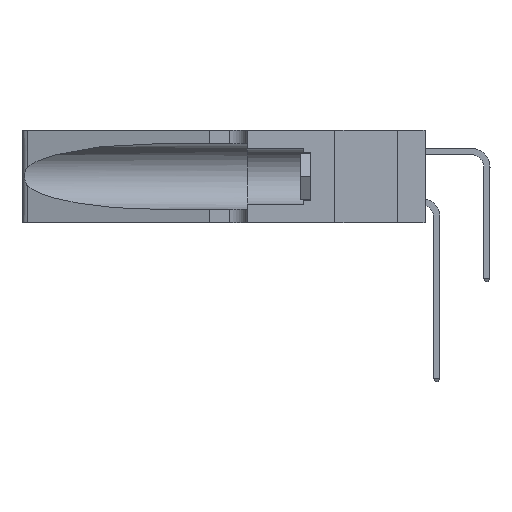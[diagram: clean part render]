
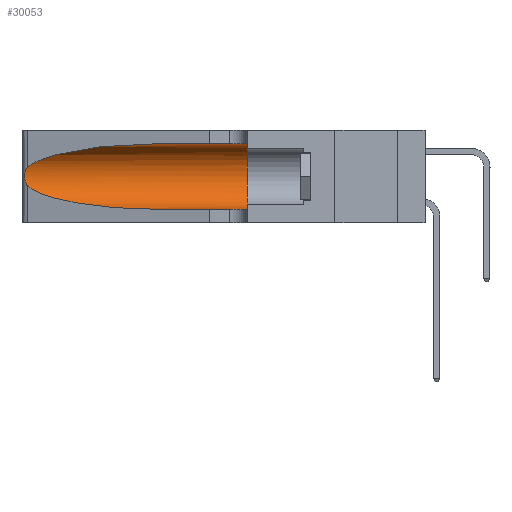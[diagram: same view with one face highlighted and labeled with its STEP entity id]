
A CAD part, left-side view. The second image highlights one B-rep face of the part: STEP entity #30053.
In plain terms, the highlighted cylindrical face has radius 3.308 mm (diameter 6.617 mm), a partial arc.
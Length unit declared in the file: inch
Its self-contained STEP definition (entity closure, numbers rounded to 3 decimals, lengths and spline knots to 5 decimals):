
#41 = ORIENTED_EDGE ( 'NONE', *, *, #12852, .T. ) ;
#842 = CARTESIAN_POINT ( 'NONE',  ( 0.2373, 1.15595, 0.08982 ) ) ;
#934 = EDGE_CURVE ( 'NONE', #26901, #13293, #1297, .T. ) ;
#1297 = LINE ( 'NONE', #4245, #10268 ) ;
#2368 = CARTESIAN_POINT ( 'NONE',  ( 0.1305, 0.35, 0.185 ) ) ;
#2374 = CARTESIAN_POINT ( 'NONE',  ( 0.25854, 1.2359, 0.20912 ) ) ;
#2505 = FACE_OUTER_BOUND ( 'NONE', #13206, .T. ) ;
#2927 = ORIENTED_EDGE ( 'NONE', *, *, #934, .T. ) ;
#3257 = CARTESIAN_POINT ( 'NONE',  ( 0.1305, 0.72297, 0.05475 ) ) ;
#4245 = CARTESIAN_POINT ( 'NONE',  ( 0.1305, 1.61858, 0.05475 ) ) ;
#4384 = CARTESIAN_POINT ( 'NONE',  ( 0.25487, 1.22718, 0.22369 ) ) ;
#4611 = CARTESIAN_POINT ( 'NONE',  ( 0.2373, 1.15595, 0.28018 ) ) ;
#4786 = CARTESIAN_POINT ( 'NONE',  ( 0.25487, 1.22718, 0.22369 ) ) ;
#4891 = EDGE_CURVE ( 'NONE', #25531, #10195, #10102, .T. ) ;
#5013 = CARTESIAN_POINT ( 'NONE',  ( 0.26018, 1.23835, 0.19895 ) ) ;
#5223 = CARTESIAN_POINT ( 'NONE',  ( 0.25487, 1.22718, 0.14631 ) ) ;
#5441 = CARTESIAN_POINT ( 'NONE',  ( 0.26017, 1.23833, 0.17102 ) ) ;
#5892 = CARTESIAN_POINT ( 'NONE',  ( 0.25487, 1.22718, 0.14631 ) ) ;
#6158 = ORIENTED_EDGE ( 'NONE', *, *, #26622, .T. ) ;
#6411 = CARTESIAN_POINT ( 'NONE',  ( 0.25487, 1.22718, 0.14631 ) ) ;
#7202 = CARTESIAN_POINT ( 'NONE',  ( 0.25555, 1.22994, 0.2215 ) ) ;
#7729 = CARTESIAN_POINT ( 'NONE',  ( 0.25856, 1.23593, 0.16098 ) ) ;
#8160 = ORIENTED_EDGE ( 'NONE', *, *, #30944, .F. ) ;
#9592 = CARTESIAN_POINT ( 'NONE',  ( 0.1305, 0.72297, 0.31525 ) ) ;
#9937 = CARTESIAN_POINT ( 'NONE',  ( 0.25487, 1.22718, 0.22369 ) ) ;
#10102 = B_SPLINE_CURVE_WITH_KNOTS ( 'NONE', 3,
 ( #4786, #7202, #12595, #30960, #2374, #5013, #21016, #23718, #5441, #7729, #25909, #18174, #10329, #5223 ),
 .UNSPECIFIED., .F., .F.,
 ( 4, 2, 2, 2, 2, 2, 4 ),
 ( 0., 0.00027, 0.00053, 0.00107, 0.0016, 0.00187, 0.00214 ),
 .UNSPECIFIED. ) ;
#10195 = VERTEX_POINT ( 'NONE', #6411 ) ;
#10268 = VECTOR ( 'NONE', #11829, 39.37008 ) ;
#10329 = CARTESIAN_POINT ( 'NONE',  ( 0.25555, 1.22993, 0.14849 ) ) ;
#11492 = DIRECTION ( 'NONE',  ( 0., -1., 0. ) ) ;
#11829 = DIRECTION ( 'NONE',  ( 0., -1., 0. ) ) ;
#12595 = CARTESIAN_POINT ( 'NONE',  ( 0.25639, 1.23184, 0.21858 ) ) ;
#12786 =( BOUNDED_CURVE ( )  B_SPLINE_CURVE ( 3, ( #9592, #17545, #4611, #9937 ),
 .UNSPECIFIED., .F., .F. ) 
 B_SPLINE_CURVE_WITH_KNOTS ( ( 4, 4 ),
 ( 1.5708, 2.84003 ),
 .UNSPECIFIED. ) 
 CURVE ( )  GEOMETRIC_REPRESENTATION_ITEM ( )  RATIONAL_B_SPLINE_CURVE ( ( 1., 0.87, 0.87, 1. ) ) 
 REPRESENTATION_ITEM ( '' )  );
#12852 = EDGE_CURVE ( 'NONE', #17965, #25531, #12786, .T. ) ;
#13135 = DIRECTION ( 'NONE',  ( 0., 1., 0. ) ) ;
#13206 = EDGE_LOOP ( 'NONE', ( #41, #30131, #6158, #2927, #8160, #27792 ) ) ;
#13293 = VERTEX_POINT ( 'NONE', #29082 ) ;
#13762 = CARTESIAN_POINT ( 'NONE',  ( 0.1305, 1.61858, 0.31525 ) ) ;
#14476 = DIRECTION ( 'NONE',  ( 0., 0., -1. ) ) ;
#16299 = CYLINDRICAL_SURFACE ( 'NONE', #29642, 0.13025 ) ;
#16380 = DIRECTION ( 'NONE',  ( 0., -1., 0. ) ) ;
#17545 = CARTESIAN_POINT ( 'NONE',  ( 0.18966, 0.96281, 0.31525 ) ) ;
#17561 = CARTESIAN_POINT ( 'NONE',  ( 0.1305, 0.72297, 0.31525 ) ) ;
#17965 = VERTEX_POINT ( 'NONE', #17561 ) ;
#18174 = CARTESIAN_POINT ( 'NONE',  ( 0.25639, 1.23186, 0.15144 ) ) ;
#18830 = CARTESIAN_POINT ( 'NONE',  ( 0.18966, 0.96281, 0.05475 ) ) ;
#19600 = CARTESIAN_POINT ( 'NONE',  ( 0.1305, 1.61858, 0.185 ) ) ;
#19978 = CIRCLE ( 'NONE', #28377, 0.13025 ) ;
#21016 = CARTESIAN_POINT ( 'NONE',  ( 0.26075, 1.23896, 0.19203 ) ) ;
#21326 = EDGE_CURVE ( 'NONE', #17965, #25485, #22509, .T. ) ;
#22509 = LINE ( 'NONE', #13762, #23311 ) ;
#23311 = VECTOR ( 'NONE', #16380, 39.37008 ) ;
#23718 = CARTESIAN_POINT ( 'NONE',  ( 0.26075, 1.23896, 0.178 ) ) ;
#25226 = CARTESIAN_POINT ( 'NONE',  ( 0.1305, 0.35, 0.31525 ) ) ;
#25485 = VERTEX_POINT ( 'NONE', #25226 ) ;
#25531 = VERTEX_POINT ( 'NONE', #4384 ) ;
#25796 = DIRECTION ( 'NONE',  ( 0., 0., 1. ) ) ;
#25909 = CARTESIAN_POINT ( 'NONE',  ( 0.25789, 1.23486, 0.15765 ) ) ;
#26622 = EDGE_CURVE ( 'NONE', #10195, #26901, #26958, .T. ) ;
#26901 = VERTEX_POINT ( 'NONE', #33182 ) ;
#26958 =( BOUNDED_CURVE ( )  B_SPLINE_CURVE ( 3, ( #5892, #842, #18830, #3257 ),
 .UNSPECIFIED., .F., .F. ) 
 B_SPLINE_CURVE_WITH_KNOTS ( ( 4, 4 ),
 ( 3.44316, 4.71239 ),
 .UNSPECIFIED. ) 
 CURVE ( )  GEOMETRIC_REPRESENTATION_ITEM ( )  RATIONAL_B_SPLINE_CURVE ( ( 1., 0.87, 0.87, 1. ) ) 
 REPRESENTATION_ITEM ( '' )  );
#27792 = ORIENTED_EDGE ( 'NONE', *, *, #21326, .F. ) ;
#28377 = AXIS2_PLACEMENT_3D ( 'NONE', #2368, #13135, #25796 ) ;
#29082 = CARTESIAN_POINT ( 'NONE',  ( 0.1305, 0.35, 0.05475 ) ) ;
#29642 = AXIS2_PLACEMENT_3D ( 'NONE', #19600, #11492, #14476 ) ;
#30053 = ADVANCED_FACE ( 'NONE', ( #2505 ), #16299, .F. ) ;
#30131 = ORIENTED_EDGE ( 'NONE', *, *, #4891, .T. ) ;
#30944 = EDGE_CURVE ( 'NONE', #25485, #13293, #19978, .T. ) ;
#30960 = CARTESIAN_POINT ( 'NONE',  ( 0.25787, 1.23484, 0.2124 ) ) ;
#33182 = CARTESIAN_POINT ( 'NONE',  ( 0.1305, 0.72297, 0.05475 ) ) ;
